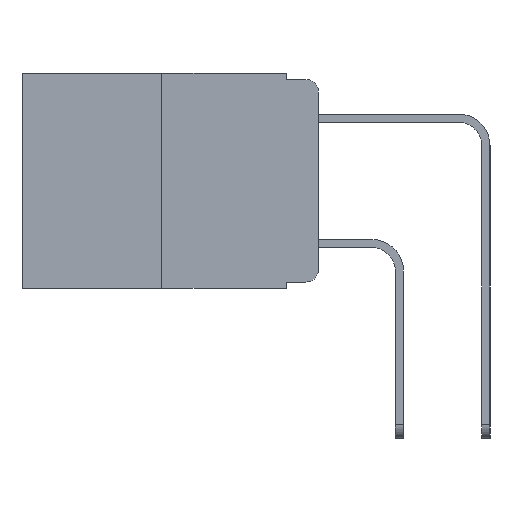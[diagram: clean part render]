
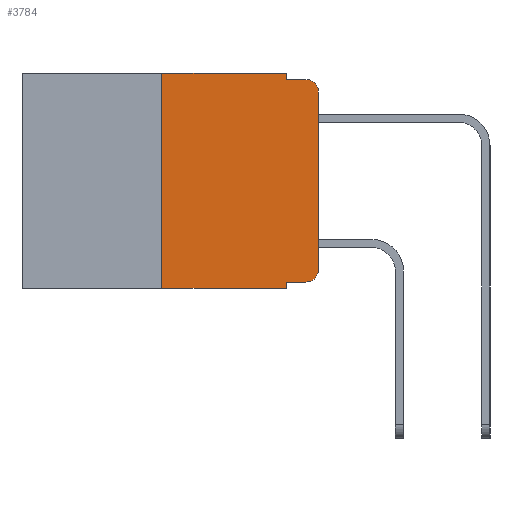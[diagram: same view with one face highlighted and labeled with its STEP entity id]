
A CAD part, left-side view. The second image highlights one B-rep face of the part: STEP entity #3784.
In plain terms, the highlighted planar face has unit normal (-1, 0, 0).
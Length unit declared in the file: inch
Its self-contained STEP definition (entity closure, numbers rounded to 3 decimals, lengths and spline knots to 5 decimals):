
#68 = DIRECTION ( 'NONE',  ( 0., 0., 1. ) ) ;
#192 = VERTEX_POINT ( 'NONE', #12365 ) ;
#624 = DIRECTION ( 'NONE',  ( 0., 0., -1. ) ) ;
#1068 = DIRECTION ( 'NONE',  ( 0., 0., -1. ) ) ;
#1172 = EDGE_CURVE ( 'NONE', #6969, #6591, #7324, .T. ) ;
#1215 = ORIENTED_EDGE ( 'NONE', *, *, #11673, .F. ) ;
#1497 = VERTEX_POINT ( 'NONE', #12582 ) ;
#1596 = AXIS2_PLACEMENT_3D ( 'NONE', #13034, #7563, #1068 ) ;
#1666 = CARTESIAN_POINT ( 'NONE',  ( 0., 0.051, 0. ) ) ;
#1853 = AXIS2_PLACEMENT_3D ( 'NONE', #8677, #2568, #9617 ) ;
#1913 = VERTEX_POINT ( 'NONE', #5653 ) ;
#2182 = ORIENTED_EDGE ( 'NONE', *, *, #1172, .T. ) ;
#2544 = ORIENTED_EDGE ( 'NONE', *, *, #8878, .T. ) ;
#2568 = DIRECTION ( 'NONE',  ( -1., 0., 0. ) ) ;
#2590 = EDGE_CURVE ( 'NONE', #6614, #3682, #7523, .T. ) ;
#2642 = CARTESIAN_POINT ( 'NONE',  ( 0., 0.02, -0.333 ) ) ;
#2670 = VECTOR ( 'NONE', #68, 39.37008 ) ;
#2702 = CARTESIAN_POINT ( 'NONE',  ( 0., 0.051, -0.01 ) ) ;
#2723 = EDGE_CURVE ( 'NONE', #3923, #6614, #8937, .T. ) ;
#3256 = LINE ( 'NONE', #1666, #10759 ) ;
#3562 = VERTEX_POINT ( 'NONE', #5843 ) ;
#3682 = VERTEX_POINT ( 'NONE', #5221 ) ;
#3784 = ADVANCED_FACE ( 'NONE', ( #12897 ), #12100, .F. ) ;
#3799 = ORIENTED_EDGE ( 'NONE', *, *, #10687, .F. ) ;
#3923 = VERTEX_POINT ( 'NONE', #9992 ) ;
#4124 = EDGE_CURVE ( 'NONE', #192, #1497, #10583, .T. ) ;
#4165 = EDGE_CURVE ( 'NONE', #1913, #8545, #7589, .T. ) ;
#4240 = EDGE_CURVE ( 'NONE', #1497, #3682, #5420, .T. ) ;
#4527 = VECTOR ( 'NONE', #7327, 39.37008 ) ;
#4603 = VECTOR ( 'NONE', #12522, 39.37008 ) ;
#5221 = CARTESIAN_POINT ( 'NONE',  ( 0., 0.02, -0.01 ) ) ;
#5311 = ORIENTED_EDGE ( 'NONE', *, *, #4165, .T. ) ;
#5420 = CIRCLE ( 'NONE', #6627, 0.02 ) ;
#5482 = CARTESIAN_POINT ( 'NONE',  ( 0., 0.051, 0. ) ) ;
#5653 = CARTESIAN_POINT ( 'NONE',  ( 0., 0.25, -0.343 ) ) ;
#5746 = LINE ( 'NONE', #10000, #10448 ) ;
#5781 = ORIENTED_EDGE ( 'NONE', *, *, #2723, .F. ) ;
#5843 = CARTESIAN_POINT ( 'NONE',  ( 0., 0.25, 0. ) ) ;
#5913 = CARTESIAN_POINT ( 'NONE',  ( 0., 0.051, -0.333 ) ) ;
#5928 = DIRECTION ( 'NONE',  ( 0., 0., 1. ) ) ;
#6109 = VECTOR ( 'NONE', #12596, 39.37008 ) ;
#6191 = DIRECTION ( 'NONE',  ( 0., -1., 0. ) ) ;
#6515 = CARTESIAN_POINT ( 'NONE',  ( 0., 0.051, -0.333 ) ) ;
#6591 = VERTEX_POINT ( 'NONE', #2642 ) ;
#6614 = VERTEX_POINT ( 'NONE', #2702 ) ;
#6627 = AXIS2_PLACEMENT_3D ( 'NONE', #12754, #7255, #624 ) ;
#6969 = VERTEX_POINT ( 'NONE', #6515 ) ;
#7017 = VECTOR ( 'NONE', #5928, 39.37008 ) ;
#7101 = EDGE_LOOP ( 'NONE', ( #9339, #7492, #12920, #5781, #1215, #11933, #5311, #3799, #2182, #2544 ) ) ;
#7255 = DIRECTION ( 'NONE',  ( -1., 0., 0. ) ) ;
#7324 = LINE ( 'NONE', #5913, #9755 ) ;
#7327 = DIRECTION ( 'NONE',  ( 0., -1., 0. ) ) ;
#7386 = CARTESIAN_POINT ( 'NONE',  ( 0., 0.051, -0.343 ) ) ;
#7492 = ORIENTED_EDGE ( 'NONE', *, *, #4240, .T. ) ;
#7523 = LINE ( 'NONE', #11266, #4527 ) ;
#7563 = DIRECTION ( 'NONE',  ( 1., 0., 0. ) ) ;
#7589 = LINE ( 'NONE', #10694, #4603 ) ;
#8116 = DIRECTION ( 'NONE',  ( 0., -1., 0. ) ) ;
#8545 = VERTEX_POINT ( 'NONE', #7386 ) ;
#8677 = CARTESIAN_POINT ( 'NONE',  ( 0., 0.02, -0.313 ) ) ;
#8878 = EDGE_CURVE ( 'NONE', #6591, #192, #12225, .T. ) ;
#8937 = LINE ( 'NONE', #5482, #6109 ) ;
#9339 = ORIENTED_EDGE ( 'NONE', *, *, #4124, .T. ) ;
#9477 = LINE ( 'NONE', #9680, #7017 ) ;
#9617 = DIRECTION ( 'NONE',  ( 0., 0., -1. ) ) ;
#9680 = CARTESIAN_POINT ( 'NONE',  ( 0., 0.25, 0. ) ) ;
#9755 = VECTOR ( 'NONE', #6191, 39.37008 ) ;
#9992 = CARTESIAN_POINT ( 'NONE',  ( 0., 0.051, 0. ) ) ;
#10000 = CARTESIAN_POINT ( 'NONE',  ( 0., 0.473, 0. ) ) ;
#10448 = VECTOR ( 'NONE', #8116, 39.37008 ) ;
#10564 = EDGE_CURVE ( 'NONE', #1913, #3562, #9477, .T. ) ;
#10583 = LINE ( 'NONE', #12396, #2670 ) ;
#10687 = EDGE_CURVE ( 'NONE', #6969, #8545, #3256, .T. ) ;
#10694 = CARTESIAN_POINT ( 'NONE',  ( 0., 0.473, -0.343 ) ) ;
#10759 = VECTOR ( 'NONE', #10760, 39.37008 ) ;
#10760 = DIRECTION ( 'NONE',  ( 0., 0., -1. ) ) ;
#11266 = CARTESIAN_POINT ( 'NONE',  ( 0., 0.051, -0.01 ) ) ;
#11673 = EDGE_CURVE ( 'NONE', #3562, #3923, #5746, .T. ) ;
#11933 = ORIENTED_EDGE ( 'NONE', *, *, #10564, .F. ) ;
#12100 = PLANE ( 'NONE',  #1596 ) ;
#12225 = CIRCLE ( 'NONE', #1853, 0.02 ) ;
#12365 = CARTESIAN_POINT ( 'NONE',  ( 0., 0., -0.313 ) ) ;
#12396 = CARTESIAN_POINT ( 'NONE',  ( 0., 0., 0. ) ) ;
#12522 = DIRECTION ( 'NONE',  ( 0., -1., 0. ) ) ;
#12582 = CARTESIAN_POINT ( 'NONE',  ( 0., 0., -0.03 ) ) ;
#12596 = DIRECTION ( 'NONE',  ( 0., 0., -1. ) ) ;
#12754 = CARTESIAN_POINT ( 'NONE',  ( 0., 0.02, -0.03 ) ) ;
#12897 = FACE_OUTER_BOUND ( 'NONE', #7101, .T. ) ;
#12920 = ORIENTED_EDGE ( 'NONE', *, *, #2590, .F. ) ;
#13034 = CARTESIAN_POINT ( 'NONE',  ( 0., 0.473, 0. ) ) ;
